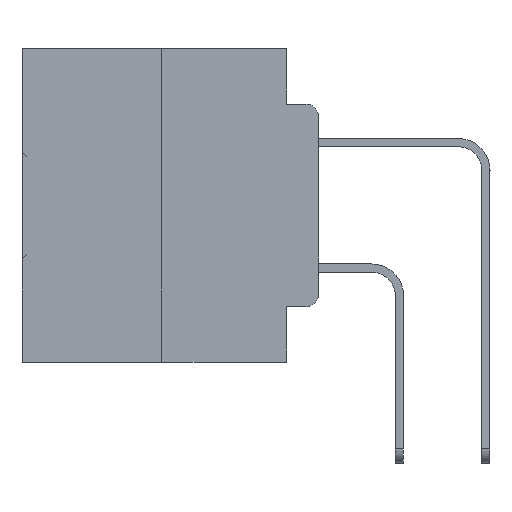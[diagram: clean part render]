
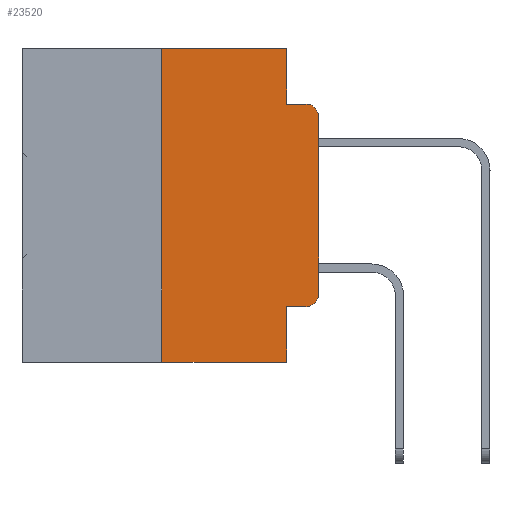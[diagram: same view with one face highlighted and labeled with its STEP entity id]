
A CAD part, left-side view. The second image highlights one B-rep face of the part: STEP entity #23520.
In plain terms, the highlighted planar face has unit normal (-1, 0, 0).
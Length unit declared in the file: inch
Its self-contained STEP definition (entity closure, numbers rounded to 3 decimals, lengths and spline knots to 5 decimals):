
#1209 = DIRECTION ( 'NONE',  ( 0., 0., -1. ) ) ;
#1485 = ORIENTED_EDGE ( 'NONE', *, *, #10011, .T. ) ;
#2074 = DIRECTION ( 'NONE',  ( 1., 0., 0. ) ) ;
#2742 = EDGE_CURVE ( 'NONE', #9598, #16811, #7804, .T. ) ;
#3890 = CARTESIAN_POINT ( 'NONE',  ( 0., 0.051, 0. ) ) ;
#4228 = CARTESIAN_POINT ( 'NONE',  ( 0., 0.051, 0. ) ) ;
#4295 = VECTOR ( 'NONE', #23421, 39.37008 ) ;
#5016 = ORIENTED_EDGE ( 'NONE', *, *, #18198, .T. ) ;
#5480 = DIRECTION ( 'NONE',  ( 0., -1., 0. ) ) ;
#5486 = CARTESIAN_POINT ( 'NONE',  ( 0., 0.051, -0.0885 ) ) ;
#5932 = CARTESIAN_POINT ( 'NONE',  ( 0., 0.02, -0.0885 ) ) ;
#5995 = VERTEX_POINT ( 'NONE', #20272 ) ;
#6165 = EDGE_CURVE ( 'NONE', #27948, #27650, #21505, .T. ) ;
#6564 = CARTESIAN_POINT ( 'NONE',  ( 0., 0., 0. ) ) ;
#6659 = CARTESIAN_POINT ( 'NONE',  ( 0., 0.051, -0.4115 ) ) ;
#6705 = DIRECTION ( 'NONE',  ( 0., 0., -1. ) ) ;
#6815 = ORIENTED_EDGE ( 'NONE', *, *, #26623, .F. ) ;
#7655 = CARTESIAN_POINT ( 'NONE',  ( 0., 0.02, -0.1085 ) ) ;
#7804 = LINE ( 'NONE', #23951, #25680 ) ;
#7924 = AXIS2_PLACEMENT_3D ( 'NONE', #15599, #2074, #6705 ) ;
#7987 = CARTESIAN_POINT ( 'NONE',  ( 0., 0.051, 0. ) ) ;
#8854 = VERTEX_POINT ( 'NONE', #6659 ) ;
#9089 = DIRECTION ( 'NONE',  ( 0., -1., 0. ) ) ;
#9110 = ORIENTED_EDGE ( 'NONE', *, *, #12365, .T. ) ;
#9173 = CIRCLE ( 'NONE', #25009, 0.02 ) ;
#9412 = LINE ( 'NONE', #6564, #4295 ) ;
#9442 = EDGE_CURVE ( 'NONE', #23117, #27650, #19321, .T. ) ;
#9598 = VERTEX_POINT ( 'NONE', #30981 ) ;
#9783 = DIRECTION ( 'NONE',  ( -1., 0., 0. ) ) ;
#10011 = EDGE_CURVE ( 'NONE', #9598, #26375, #33058, .T. ) ;
#10896 = CARTESIAN_POINT ( 'NONE',  ( 0., 0.02, -0.3915 ) ) ;
#12117 = CARTESIAN_POINT ( 'NONE',  ( 0., 0.473, 0. ) ) ;
#12273 = LINE ( 'NONE', #23102, #30117 ) ;
#12365 = EDGE_CURVE ( 'NONE', #8854, #16380, #12273, .T. ) ;
#12587 = CARTESIAN_POINT ( 'NONE',  ( 0., 0.25, 0. ) ) ;
#13905 = EDGE_CURVE ( 'NONE', #8854, #26375, #32265, .T. ) ;
#14492 = CARTESIAN_POINT ( 'NONE',  ( 0., 0.473, -0.5 ) ) ;
#15599 = CARTESIAN_POINT ( 'NONE',  ( 0., 0.473, 0. ) ) ;
#16380 = VERTEX_POINT ( 'NONE', #33698 ) ;
#16811 = VERTEX_POINT ( 'NONE', #12587 ) ;
#17226 = VECTOR ( 'NONE', #31748, 39.37008 ) ;
#18198 = EDGE_CURVE ( 'NONE', #5995, #27948, #9412, .T. ) ;
#18660 = VECTOR ( 'NONE', #30418, 39.37008 ) ;
#19182 = EDGE_LOOP ( 'NONE', ( #5016, #25258, #21689, #6815, #24456, #19582, #1485, #21539, #9110, #20820 ) ) ;
#19321 = LINE ( 'NONE', #29765, #26055 ) ;
#19582 = ORIENTED_EDGE ( 'NONE', *, *, #2742, .F. ) ;
#20099 = DIRECTION ( 'NONE',  ( 0., -1., 0. ) ) ;
#20272 = CARTESIAN_POINT ( 'NONE',  ( 0., 0., -0.3915 ) ) ;
#20761 = LINE ( 'NONE', #12117, #20873 ) ;
#20820 = ORIENTED_EDGE ( 'NONE', *, *, #24097, .T. ) ;
#20873 = VECTOR ( 'NONE', #9089, 39.37008 ) ;
#21318 = DIRECTION ( 'NONE',  ( 0., 0., 1. ) ) ;
#21505 = CIRCLE ( 'NONE', #34449, 0.02 ) ;
#21539 = ORIENTED_EDGE ( 'NONE', *, *, #13905, .F. ) ;
#21689 = ORIENTED_EDGE ( 'NONE', *, *, #9442, .F. ) ;
#23102 = CARTESIAN_POINT ( 'NONE',  ( 0., 0.051, -0.4115 ) ) ;
#23117 = VERTEX_POINT ( 'NONE', #5486 ) ;
#23209 = FACE_OUTER_BOUND ( 'NONE', #19182, .T. ) ;
#23421 = DIRECTION ( 'NONE',  ( 0., 0., 1. ) ) ;
#23520 = ADVANCED_FACE ( 'NONE', ( #23209 ), #28676, .F. ) ;
#23805 = DIRECTION ( 'NONE',  ( 0., 0., -1. ) ) ;
#23951 = CARTESIAN_POINT ( 'NONE',  ( 0., 0.25, 0. ) ) ;
#24097 = EDGE_CURVE ( 'NONE', #16380, #5995, #9173, .T. ) ;
#24456 = ORIENTED_EDGE ( 'NONE', *, *, #33707, .F. ) ;
#25009 = AXIS2_PLACEMENT_3D ( 'NONE', #10896, #32510, #32161 ) ;
#25258 = ORIENTED_EDGE ( 'NONE', *, *, #6165, .T. ) ;
#25680 = VECTOR ( 'NONE', #21318, 39.37008 ) ;
#26055 = VECTOR ( 'NONE', #5480, 39.37008 ) ;
#26375 = VERTEX_POINT ( 'NONE', #31914 ) ;
#26623 = EDGE_CURVE ( 'NONE', #28624, #23117, #28517, .T. ) ;
#27650 = VERTEX_POINT ( 'NONE', #5932 ) ;
#27948 = VERTEX_POINT ( 'NONE', #31780 ) ;
#28517 = LINE ( 'NONE', #4228, #30707 ) ;
#28624 = VERTEX_POINT ( 'NONE', #3890 ) ;
#28676 = PLANE ( 'NONE',  #7924 ) ;
#29765 = CARTESIAN_POINT ( 'NONE',  ( 0., 0.051, -0.0885 ) ) ;
#30117 = VECTOR ( 'NONE', #20099, 39.37008 ) ;
#30418 = DIRECTION ( 'NONE',  ( 0., -1., 0. ) ) ;
#30707 = VECTOR ( 'NONE', #1209, 39.37008 ) ;
#30981 = CARTESIAN_POINT ( 'NONE',  ( 0., 0.25, -0.5 ) ) ;
#31748 = DIRECTION ( 'NONE',  ( 0., 0., -1. ) ) ;
#31780 = CARTESIAN_POINT ( 'NONE',  ( 0., 0., -0.1085 ) ) ;
#31914 = CARTESIAN_POINT ( 'NONE',  ( 0., 0.051, -0.5 ) ) ;
#32161 = DIRECTION ( 'NONE',  ( 0., 0., -1. ) ) ;
#32265 = LINE ( 'NONE', #7987, #17226 ) ;
#32510 = DIRECTION ( 'NONE',  ( -1., 0., 0. ) ) ;
#33058 = LINE ( 'NONE', #14492, #18660 ) ;
#33698 = CARTESIAN_POINT ( 'NONE',  ( 0., 0.02, -0.4115 ) ) ;
#33707 = EDGE_CURVE ( 'NONE', #16811, #28624, #20761, .T. ) ;
#34449 = AXIS2_PLACEMENT_3D ( 'NONE', #7655, #9783, #23805 ) ;
